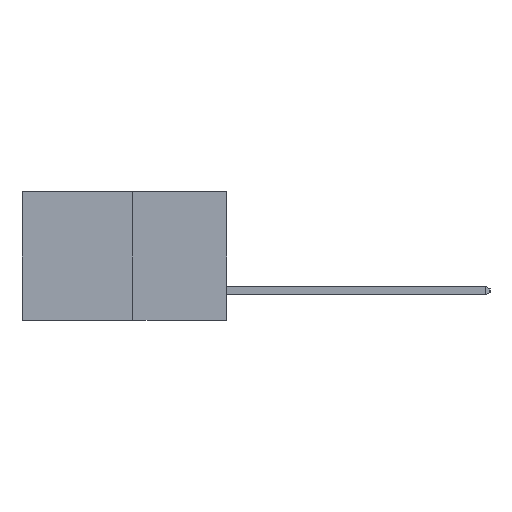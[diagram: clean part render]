
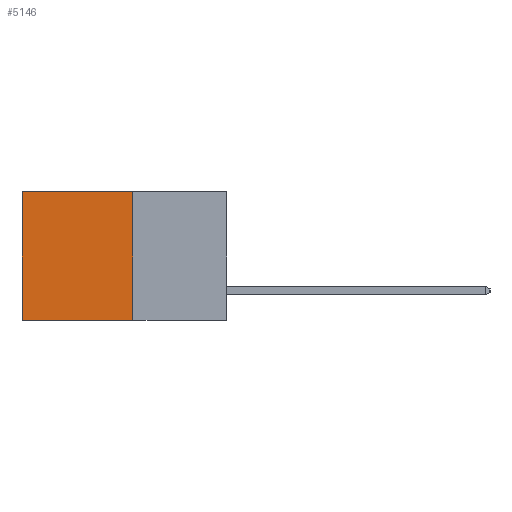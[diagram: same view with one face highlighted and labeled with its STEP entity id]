
A CAD part, left-side view. The second image highlights one B-rep face of the part: STEP entity #5146.
In plain terms, the highlighted planar face has unit normal (-1, 0, 0).
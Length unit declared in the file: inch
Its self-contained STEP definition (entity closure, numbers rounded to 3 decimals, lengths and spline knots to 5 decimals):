
#579 = EDGE_CURVE ( 'NONE', #7118, #11148, #5153, .T. ) ;
#1106 = AXIS2_PLACEMENT_3D ( 'NONE', #3315, #16190, #5187 ) ;
#1198 = CARTESIAN_POINT ( 'NONE',  ( 0.277, 0.59, -0.37 ) ) ;
#1289 = CARTESIAN_POINT ( 'NONE',  ( 0.277, 0.59, -0.37 ) ) ;
#3315 = CARTESIAN_POINT ( 'NONE',  ( 0.277, 0.27, -0.37 ) ) ;
#3644 = CARTESIAN_POINT ( 'NONE',  ( 0.277, 0.27, -0.37 ) ) ;
#3831 = VECTOR ( 'NONE', #18880, 39.37008 ) ;
#5146 = ADVANCED_FACE ( 'NONE', ( #6790 ), #14342, .F. ) ;
#5153 = LINE ( 'NONE', #9369, #9465 ) ;
#5187 = DIRECTION ( 'NONE',  ( 0., 0., -1. ) ) ;
#5997 = CARTESIAN_POINT ( 'NONE',  ( 0.277, 0.27, 0. ) ) ;
#6790 = FACE_OUTER_BOUND ( 'NONE', #19926, .T. ) ;
#7118 = VERTEX_POINT ( 'NONE', #10392 ) ;
#7806 = LINE ( 'NONE', #1289, #16427 ) ;
#9134 = ORIENTED_EDGE ( 'NONE', *, *, #11316, .T. ) ;
#9369 = CARTESIAN_POINT ( 'NONE',  ( 0.277, 0.27, -0.37 ) ) ;
#9465 = VECTOR ( 'NONE', #10288, 39.37008 ) ;
#9657 = CARTESIAN_POINT ( 'NONE',  ( 0.277, 0.59, 0. ) ) ;
#10288 = DIRECTION ( 'NONE',  ( 0., 0., -1. ) ) ;
#10392 = CARTESIAN_POINT ( 'NONE',  ( 0.277, 0.27, 0. ) ) ;
#10434 = ORIENTED_EDGE ( 'NONE', *, *, #579, .F. ) ;
#10566 = CARTESIAN_POINT ( 'NONE',  ( 0.277, 0.27, -0.37 ) ) ;
#10960 = VERTEX_POINT ( 'NONE', #1198 ) ;
#11148 = VERTEX_POINT ( 'NONE', #3644 ) ;
#11316 = EDGE_CURVE ( 'NONE', #7118, #18206, #17947, .T. ) ;
#11628 = EDGE_CURVE ( 'NONE', #11148, #10960, #16480, .T. ) ;
#12404 = DIRECTION ( 'NONE',  ( 0., 1., 0. ) ) ;
#14113 = ORIENTED_EDGE ( 'NONE', *, *, #20571, .T. ) ;
#14342 = PLANE ( 'NONE',  #1106 ) ;
#16190 = DIRECTION ( 'NONE',  ( 1., 0., 0. ) ) ;
#16427 = VECTOR ( 'NONE', #23424, 39.37008 ) ;
#16480 = LINE ( 'NONE', #10566, #20223 ) ;
#16858 = ORIENTED_EDGE ( 'NONE', *, *, #11628, .F. ) ;
#17947 = LINE ( 'NONE', #5997, #3831 ) ;
#18206 = VERTEX_POINT ( 'NONE', #9657 ) ;
#18880 = DIRECTION ( 'NONE',  ( 0., 1., 0. ) ) ;
#19926 = EDGE_LOOP ( 'NONE', ( #14113, #16858, #10434, #9134 ) ) ;
#20223 = VECTOR ( 'NONE', #12404, 39.37008 ) ;
#20571 = EDGE_CURVE ( 'NONE', #18206, #10960, #7806, .T. ) ;
#23424 = DIRECTION ( 'NONE',  ( 0., 0., -1. ) ) ;
